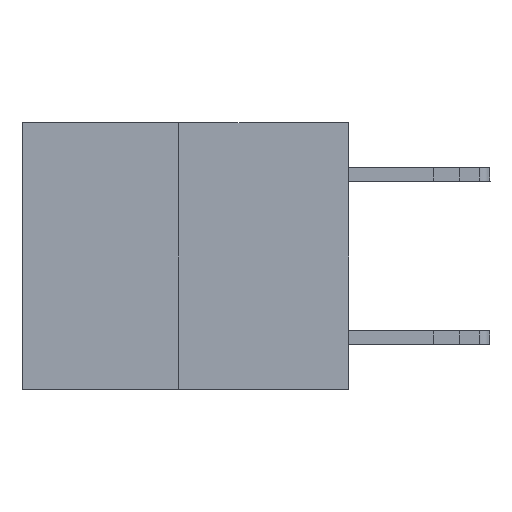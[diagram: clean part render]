
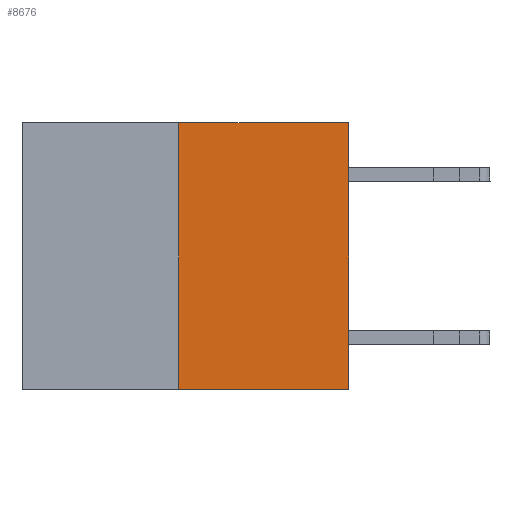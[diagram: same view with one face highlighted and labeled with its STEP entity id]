
A CAD part, left-side view. The second image highlights one B-rep face of the part: STEP entity #8676.
In plain terms, the highlighted planar face has unit normal (-1, 0, 0).
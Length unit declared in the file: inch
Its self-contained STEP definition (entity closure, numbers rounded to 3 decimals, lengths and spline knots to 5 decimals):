
#1139 = VECTOR ( 'NONE', #5647, 39.37008 ) ;
#1923 = DIRECTION ( 'NONE',  ( 0., -1., 0. ) ) ;
#2704 = DIRECTION ( 'NONE',  ( 1., 0., 0. ) ) ;
#2732 = EDGE_CURVE ( 'NONE', #28121, #9452, #6114, .T. ) ;
#5647 = DIRECTION ( 'NONE',  ( 0., -1., 0. ) ) ;
#5908 = ORIENTED_EDGE ( 'NONE', *, *, #10489, .T. ) ;
#6114 = LINE ( 'NONE', #25743, #1139 ) ;
#6437 = EDGE_CURVE ( 'NONE', #28121, #28781, #21003, .T. ) ;
#7644 = PLANE ( 'NONE',  #13951 ) ;
#7887 = CARTESIAN_POINT ( 'NONE',  ( 0., 0.312, -0.49 ) ) ;
#8676 = ADVANCED_FACE ( 'NONE', ( #26163 ), #7644, .F. ) ;
#8995 = CARTESIAN_POINT ( 'NONE',  ( 0., 0.312, 0. ) ) ;
#9412 = DIRECTION ( 'NONE',  ( 0., 0., -1. ) ) ;
#9452 = VERTEX_POINT ( 'NONE', #16237 ) ;
#10489 = EDGE_CURVE ( 'NONE', #9452, #24249, #25363, .T. ) ;
#13951 = AXIS2_PLACEMENT_3D ( 'NONE', #20753, #2704, #9412 ) ;
#15480 = ORIENTED_EDGE ( 'NONE', *, *, #6437, .F. ) ;
#15485 = CARTESIAN_POINT ( 'NONE',  ( 0., 0.6, 0. ) ) ;
#16083 = EDGE_LOOP ( 'NONE', ( #15480, #18577, #5908, #24058 ) ) ;
#16237 = CARTESIAN_POINT ( 'NONE',  ( 0., 0., -0.49 ) ) ;
#16788 = LINE ( 'NONE', #15485, #20643 ) ;
#17680 = CARTESIAN_POINT ( 'NONE',  ( 0., 0.312, -0.49 ) ) ;
#17958 = DIRECTION ( 'NONE',  ( 0., 0., 1. ) ) ;
#18577 = ORIENTED_EDGE ( 'NONE', *, *, #2732, .T. ) ;
#19561 = CARTESIAN_POINT ( 'NONE',  ( 0., 0., 0. ) ) ;
#20061 = VECTOR ( 'NONE', #23993, 39.37008 ) ;
#20430 = EDGE_CURVE ( 'NONE', #28781, #24249, #16788, .T. ) ;
#20643 = VECTOR ( 'NONE', #1923, 39.37008 ) ;
#20753 = CARTESIAN_POINT ( 'NONE',  ( 0., 0.6, 0. ) ) ;
#21003 = LINE ( 'NONE', #17680, #24488 ) ;
#23993 = DIRECTION ( 'NONE',  ( 0., 0., 1. ) ) ;
#24058 = ORIENTED_EDGE ( 'NONE', *, *, #20430, .F. ) ;
#24249 = VERTEX_POINT ( 'NONE', #28177 ) ;
#24488 = VECTOR ( 'NONE', #17958, 39.37008 ) ;
#25363 = LINE ( 'NONE', #19561, #20061 ) ;
#25743 = CARTESIAN_POINT ( 'NONE',  ( 0., 0.6, -0.49 ) ) ;
#26163 = FACE_OUTER_BOUND ( 'NONE', #16083, .T. ) ;
#28121 = VERTEX_POINT ( 'NONE', #7887 ) ;
#28177 = CARTESIAN_POINT ( 'NONE',  ( 0., 0., 0. ) ) ;
#28781 = VERTEX_POINT ( 'NONE', #8995 ) ;
